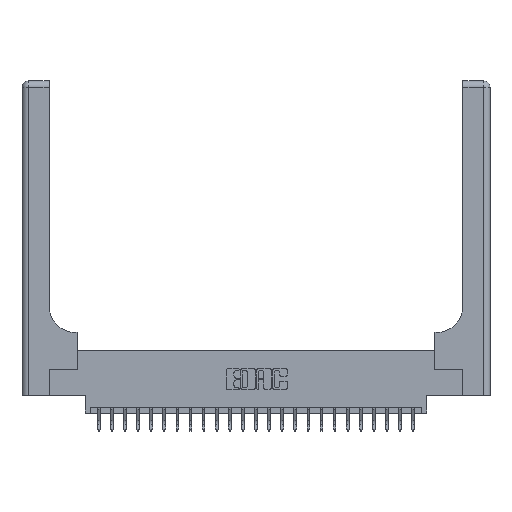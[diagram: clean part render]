
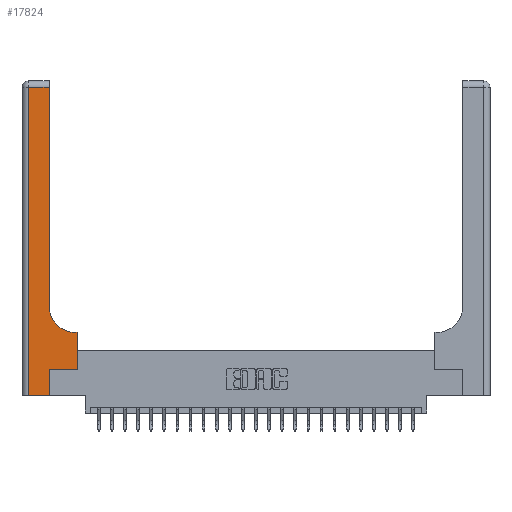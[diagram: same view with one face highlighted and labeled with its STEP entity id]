
A CAD part, top view. The second image highlights one B-rep face of the part: STEP entity #17824.
In plain terms, the highlighted planar face has unit normal (0, 0, 1).
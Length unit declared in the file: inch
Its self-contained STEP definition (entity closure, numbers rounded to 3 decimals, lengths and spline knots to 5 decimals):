
#764 = CARTESIAN_POINT ( 'NONE',  ( 0.26, 3., 0.37 ) ) ;
#1944 = EDGE_CURVE ( 'NONE', #22576, #10049, #23435, .T. ) ;
#2399 = ORIENTED_EDGE ( 'NONE', *, *, #12885, .T. ) ;
#2401 = ORIENTED_EDGE ( 'NONE', *, *, #7124, .T. ) ;
#2668 = CARTESIAN_POINT ( 'NONE',  ( 0.265, 0.25, 0.37 ) ) ;
#2760 = EDGE_CURVE ( 'NONE', #6217, #15082, #10657, .T. ) ;
#2780 = ORIENTED_EDGE ( 'NONE', *, *, #3656, .T. ) ;
#2989 = VECTOR ( 'NONE', #19545, 39.37008 ) ;
#2992 = VECTOR ( 'NONE', #17178, 39.37008 ) ;
#3031 = LINE ( 'NONE', #8655, #11797 ) ;
#3238 = PLANE ( 'NONE',  #9089 ) ;
#3656 = EDGE_CURVE ( 'NONE', #17299, #22639, #4358, .T. ) ;
#3671 = ORIENTED_EDGE ( 'NONE', *, *, #12668, .T. ) ;
#4319 = VERTEX_POINT ( 'NONE', #8809 ) ;
#4358 = LINE ( 'NONE', #10346, #2989 ) ;
#4433 = EDGE_CURVE ( 'NONE', #12092, #6217, #13629, .T. ) ;
#4483 = VECTOR ( 'NONE', #24455, 39.37008 ) ;
#4537 = CARTESIAN_POINT ( 'NONE',  ( 0., 0., 0.37 ) ) ;
#4597 = DIRECTION ( 'NONE',  ( 0., 0., -1. ) ) ;
#4962 = DIRECTION ( 'NONE',  ( 0., 0., -1. ) ) ;
#6088 = ORIENTED_EDGE ( 'NONE', *, *, #1944, .T. ) ;
#6217 = VERTEX_POINT ( 'NONE', #11737 ) ;
#6454 = VECTOR ( 'NONE', #15751, 39.37008 ) ;
#6503 = CARTESIAN_POINT ( 'NONE',  ( 0.528, 0.6, 0.37 ) ) ;
#7028 = CIRCLE ( 'NONE', #20939, 0.25 ) ;
#7124 = EDGE_CURVE ( 'NONE', #13024, #12092, #17863, .T. ) ;
#7155 = VECTOR ( 'NONE', #17948, 39.37008 ) ;
#7303 = CARTESIAN_POINT ( 'NONE',  ( 0.265, 0., 0.37 ) ) ;
#7619 = CARTESIAN_POINT ( 'NONE',  ( 0.26, 2.94, 0.37 ) ) ;
#7715 = DIRECTION ( 'NONE',  ( 0., -1., 0. ) ) ;
#7974 = ORIENTED_EDGE ( 'NONE', *, *, #13896, .T. ) ;
#8467 = CARTESIAN_POINT ( 'NONE',  ( 0.51, 0.85, 0.37 ) ) ;
#8582 = VECTOR ( 'NONE', #7715, 39.37008 ) ;
#8655 = CARTESIAN_POINT ( 'NONE',  ( 0.528, 0.25, 0.37 ) ) ;
#8809 = CARTESIAN_POINT ( 'NONE',  ( 0.06, 2.94, 0.37 ) ) ;
#9089 = AXIS2_PLACEMENT_3D ( 'NONE', #10843, #4597, #18426 ) ;
#9421 = CARTESIAN_POINT ( 'NONE',  ( 0.528, 0.25, 0.37 ) ) ;
#10049 = VERTEX_POINT ( 'NONE', #7619 ) ;
#10346 = CARTESIAN_POINT ( 'NONE',  ( 0.26, 0.6, 0.37 ) ) ;
#10657 = LINE ( 'NONE', #2668, #15519 ) ;
#10843 = CARTESIAN_POINT ( 'NONE',  ( 0., 3., 0.37 ) ) ;
#11100 = CARTESIAN_POINT ( 'NONE',  ( 0., 2.94, 0.37 ) ) ;
#11737 = CARTESIAN_POINT ( 'NONE',  ( 0.265, 0.25, 0.37 ) ) ;
#11797 = VECTOR ( 'NONE', #23584, 39.37008 ) ;
#12092 = VERTEX_POINT ( 'NONE', #7303 ) ;
#12570 = FACE_OUTER_BOUND ( 'NONE', #20262, .T. ) ;
#12668 = EDGE_CURVE ( 'NONE', #10049, #4319, #16807, .T. ) ;
#12885 = EDGE_CURVE ( 'NONE', #4319, #13024, #13811, .T. ) ;
#13024 = VERTEX_POINT ( 'NONE', #21892 ) ;
#13629 = LINE ( 'NONE', #22970, #4483 ) ;
#13811 = LINE ( 'NONE', #21399, #8582 ) ;
#13896 = EDGE_CURVE ( 'NONE', #15082, #17299, #3031, .T. ) ;
#14320 = EDGE_CURVE ( 'NONE', #22639, #22576, #7028, .T. ) ;
#15082 = VERTEX_POINT ( 'NONE', #9421 ) ;
#15519 = VECTOR ( 'NONE', #23843, 39.37008 ) ;
#15751 = DIRECTION ( 'NONE',  ( 1., 0., 0. ) ) ;
#16807 = LINE ( 'NONE', #11100, #2992 ) ;
#17154 = ORIENTED_EDGE ( 'NONE', *, *, #4433, .T. ) ;
#17178 = DIRECTION ( 'NONE',  ( -1., 0., 0. ) ) ;
#17256 = CARTESIAN_POINT ( 'NONE',  ( 0.26, 0.85, 0.37 ) ) ;
#17299 = VERTEX_POINT ( 'NONE', #6503 ) ;
#17824 = ADVANCED_FACE ( 'NONE', ( #12570 ), #3238, .F. ) ;
#17863 = LINE ( 'NONE', #4537, #6454 ) ;
#17948 = DIRECTION ( 'NONE',  ( 0., 1., 0. ) ) ;
#18298 = DIRECTION ( 'NONE',  ( 1., 0., 0. ) ) ;
#18426 = DIRECTION ( 'NONE',  ( -1., 0., 0. ) ) ;
#19545 = DIRECTION ( 'NONE',  ( -1., 0., 0. ) ) ;
#20262 = EDGE_LOOP ( 'NONE', ( #6088, #3671, #2399, #2401, #17154, #22051, #7974, #2780, #22019 ) ) ;
#20939 = AXIS2_PLACEMENT_3D ( 'NONE', #8467, #4962, #18298 ) ;
#20985 = CARTESIAN_POINT ( 'NONE',  ( 0.51, 0.6, 0.37 ) ) ;
#21399 = CARTESIAN_POINT ( 'NONE',  ( 0.06, 3., 0.37 ) ) ;
#21892 = CARTESIAN_POINT ( 'NONE',  ( 0.06, 0., 0.37 ) ) ;
#22019 = ORIENTED_EDGE ( 'NONE', *, *, #14320, .T. ) ;
#22051 = ORIENTED_EDGE ( 'NONE', *, *, #2760, .T. ) ;
#22576 = VERTEX_POINT ( 'NONE', #17256 ) ;
#22639 = VERTEX_POINT ( 'NONE', #20985 ) ;
#22970 = CARTESIAN_POINT ( 'NONE',  ( 0.265, 0., 0.37 ) ) ;
#23435 = LINE ( 'NONE', #764, #7155 ) ;
#23584 = DIRECTION ( 'NONE',  ( 0., 1., 0. ) ) ;
#23843 = DIRECTION ( 'NONE',  ( 1., 0., 0. ) ) ;
#24455 = DIRECTION ( 'NONE',  ( 0., 1., 0. ) ) ;
